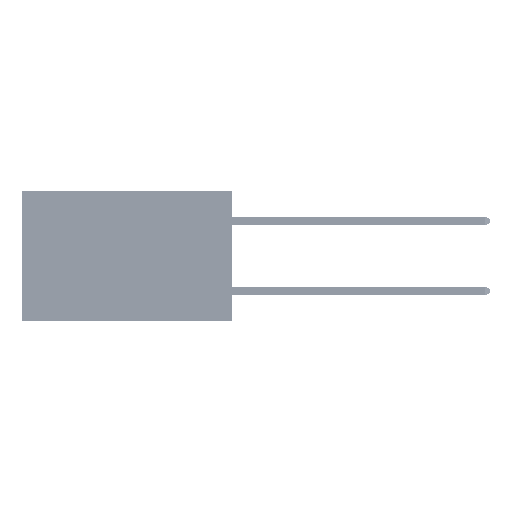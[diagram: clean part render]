
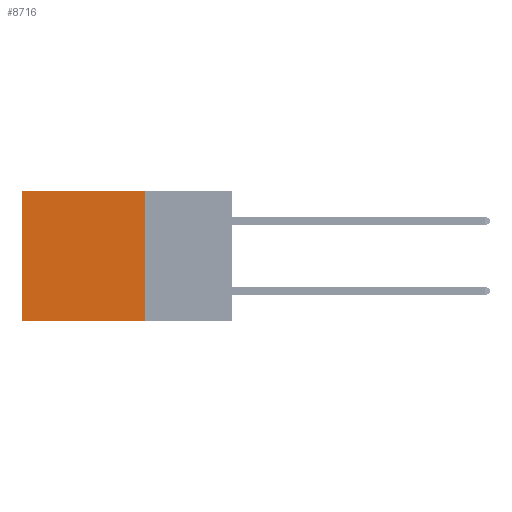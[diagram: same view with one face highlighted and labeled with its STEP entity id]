
A CAD part, left-side view. The second image highlights one B-rep face of the part: STEP entity #8716.
In plain terms, the highlighted planar face has unit normal (-1, 0, 0).
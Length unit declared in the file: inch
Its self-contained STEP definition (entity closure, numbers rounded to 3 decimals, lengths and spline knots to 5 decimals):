
#2734 = VERTEX_POINT ( 'NONE', #43131 ) ;
#3851 = VECTOR ( 'NONE', #39479, 39.37008 ) ;
#4196 = DIRECTION ( 'NONE',  ( 0., 1., 0. ) ) ;
#5933 = DIRECTION ( 'NONE',  ( 0., 0., -1. ) ) ;
#7488 = CARTESIAN_POINT ( 'NONE',  ( 0.2875, 0.25, 0. ) ) ;
#8716 = ADVANCED_FACE ( 'NONE', ( #40220 ), #32343, .F. ) ;
#8998 = CARTESIAN_POINT ( 'NONE',  ( 0.2875, 0.25, 0. ) ) ;
#9738 = VECTOR ( 'NONE', #29573, 39.37008 ) ;
#10310 = LINE ( 'NONE', #14686, #9738 ) ;
#12137 = LINE ( 'NONE', #27335, #3851 ) ;
#12583 = EDGE_CURVE ( 'NONE', #21786, #40744, #17290, .T. ) ;
#14686 = CARTESIAN_POINT ( 'NONE',  ( 0.2875, 0.25, -0.37 ) ) ;
#17290 = LINE ( 'NONE', #7488, #37861 ) ;
#21786 = VERTEX_POINT ( 'NONE', #8998 ) ;
#25742 = EDGE_CURVE ( 'NONE', #40744, #48514, #12137, .T. ) ;
#26043 = EDGE_CURVE ( 'NONE', #2734, #48514, #10310, .T. ) ;
#27335 = CARTESIAN_POINT ( 'NONE',  ( 0.2875, 0.6, 0. ) ) ;
#28144 = CARTESIAN_POINT ( 'NONE',  ( 0.2875, 0.6, -0.37 ) ) ;
#28775 = AXIS2_PLACEMENT_3D ( 'NONE', #40390, #47931, #44004 ) ;
#29573 = DIRECTION ( 'NONE',  ( 0., 1., 0. ) ) ;
#32343 = PLANE ( 'NONE',  #28775 ) ;
#34611 = CARTESIAN_POINT ( 'NONE',  ( 0.2875, 0.6, 0. ) ) ;
#34684 = LINE ( 'NONE', #46939, #42327 ) ;
#35380 = ORIENTED_EDGE ( 'NONE', *, *, #26043, .F. ) ;
#35422 = ORIENTED_EDGE ( 'NONE', *, *, #12583, .T. ) ;
#37535 = EDGE_LOOP ( 'NONE', ( #43613, #35380, #39246, #35422 ) ) ;
#37861 = VECTOR ( 'NONE', #4196, 39.37008 ) ;
#39246 = ORIENTED_EDGE ( 'NONE', *, *, #43682, .F. ) ;
#39479 = DIRECTION ( 'NONE',  ( 0., 0., -1. ) ) ;
#40220 = FACE_OUTER_BOUND ( 'NONE', #37535, .T. ) ;
#40390 = CARTESIAN_POINT ( 'NONE',  ( 0.2875, 0.25, 0. ) ) ;
#40744 = VERTEX_POINT ( 'NONE', #34611 ) ;
#42327 = VECTOR ( 'NONE', #5933, 39.37008 ) ;
#43131 = CARTESIAN_POINT ( 'NONE',  ( 0.2875, 0.25, -0.37 ) ) ;
#43613 = ORIENTED_EDGE ( 'NONE', *, *, #25742, .T. ) ;
#43682 = EDGE_CURVE ( 'NONE', #21786, #2734, #34684, .T. ) ;
#44004 = DIRECTION ( 'NONE',  ( 0., 0., -1. ) ) ;
#46939 = CARTESIAN_POINT ( 'NONE',  ( 0.2875, 0.25, 0. ) ) ;
#47931 = DIRECTION ( 'NONE',  ( 1., 0., 0. ) ) ;
#48514 = VERTEX_POINT ( 'NONE', #28144 ) ;
